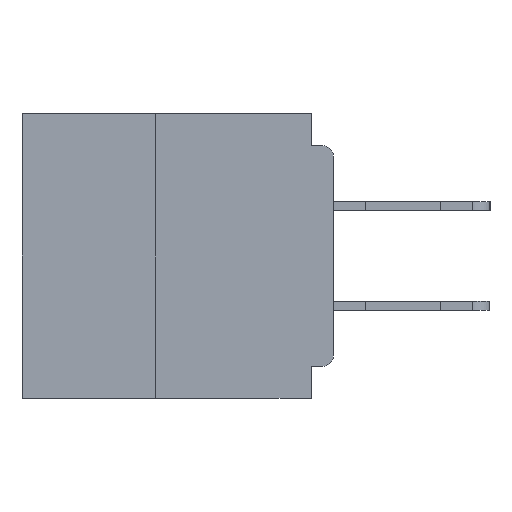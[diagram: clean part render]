
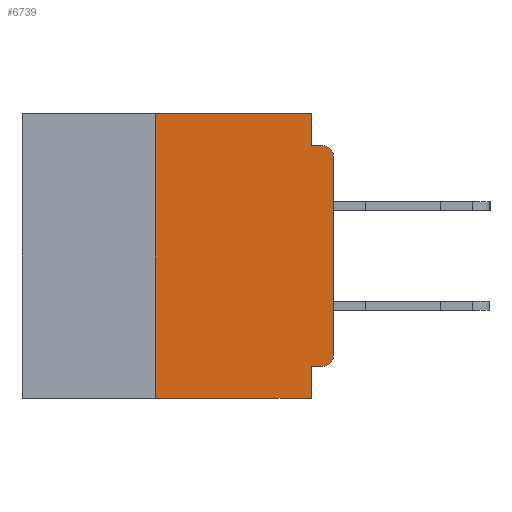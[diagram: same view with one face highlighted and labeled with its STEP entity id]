
A CAD part, left-side view. The second image highlights one B-rep face of the part: STEP entity #6739.
In plain terms, the highlighted planar face has unit normal (-1, 0, 0).
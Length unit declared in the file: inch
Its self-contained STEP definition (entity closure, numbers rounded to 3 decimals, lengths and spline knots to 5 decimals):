
#289 = AXIS2_PLACEMENT_3D ( 'NONE', #23680, #23636, #23599 ) ;
#902 = EDGE_CURVE ( 'NONE', #31502, #34823, #28456, .T. ) ;
#967 = DIRECTION ( 'NONE',  ( 0., -1., 0. ) ) ;
#1004 = FACE_OUTER_BOUND ( 'NONE', #19015, .T. ) ;
#1348 = EDGE_CURVE ( 'NONE', #32231, #15883, #28927, .T. ) ;
#1712 = ORIENTED_EDGE ( 'NONE', *, *, #23833, .F. ) ;
#2177 = LINE ( 'NONE', #33978, #9064 ) ;
#2724 = CARTESIAN_POINT ( 'NONE',  ( 0., 0.015, -0.355 ) ) ;
#2748 = VECTOR ( 'NONE', #9800, 39.37008 ) ;
#3122 = CARTESIAN_POINT ( 'NONE',  ( 0., 0.031, -0.045 ) ) ;
#3628 = EDGE_CURVE ( 'NONE', #30829, #5075, #4797, .T. ) ;
#3635 = VERTEX_POINT ( 'NONE', #24005 ) ;
#3698 = CARTESIAN_POINT ( 'NONE',  ( 0., 0.437, 0. ) ) ;
#3938 = CARTESIAN_POINT ( 'NONE',  ( 0., 0., -0.045 ) ) ;
#4179 = CIRCLE ( 'NONE', #33812, 0.015 ) ;
#4310 = EDGE_CURVE ( 'NONE', #5075, #3635, #10366, .T. ) ;
#4797 = CIRCLE ( 'NONE', #289, 0.015 ) ;
#5075 = VERTEX_POINT ( 'NONE', #13107 ) ;
#5424 = CARTESIAN_POINT ( 'NONE',  ( 0., 0.25, -0.4 ) ) ;
#5605 = DIRECTION ( 'NONE',  ( -1., 0., 0. ) ) ;
#5881 = VECTOR ( 'NONE', #26564, 39.37008 ) ;
#6739 = ADVANCED_FACE ( 'NONE', ( #1004 ), #11468, .F. ) ;
#8107 = VERTEX_POINT ( 'NONE', #34473 ) ;
#8190 = DIRECTION ( 'NONE',  ( 0., 1., 0. ) ) ;
#8366 = DIRECTION ( 'NONE',  ( 0., 0., 1. ) ) ;
#8437 = CARTESIAN_POINT ( 'NONE',  ( 0., 0.25, -0.4 ) ) ;
#8696 = DIRECTION ( 'NONE',  ( 0., 0., 1. ) ) ;
#9035 = CARTESIAN_POINT ( 'NONE',  ( 0., 0., 0. ) ) ;
#9064 = VECTOR ( 'NONE', #11214, 39.37008 ) ;
#9800 = DIRECTION ( 'NONE',  ( 0., -1., 0. ) ) ;
#10366 = LINE ( 'NONE', #9035, #11311 ) ;
#10683 = AXIS2_PLACEMENT_3D ( 'NONE', #11421, #11381, #11342 ) ;
#11214 = DIRECTION ( 'NONE',  ( 0., 0., -1. ) ) ;
#11311 = VECTOR ( 'NONE', #8696, 39.37008 ) ;
#11342 = DIRECTION ( 'NONE',  ( 0., 0., -1. ) ) ;
#11381 = DIRECTION ( 'NONE',  ( 1., 0., 0. ) ) ;
#11421 = CARTESIAN_POINT ( 'NONE',  ( 0., 0.437, 0. ) ) ;
#11468 = PLANE ( 'NONE',  #10683 ) ;
#11872 = EDGE_CURVE ( 'NONE', #3635, #8107, #4179, .T. ) ;
#12154 = VERTEX_POINT ( 'NONE', #24176 ) ;
#12159 = EDGE_CURVE ( 'NONE', #15883, #8107, #18328, .T. ) ;
#12610 = VECTOR ( 'NONE', #8366, 39.37008 ) ;
#13107 = CARTESIAN_POINT ( 'NONE',  ( 0., 0., -0.34 ) ) ;
#14173 = VERTEX_POINT ( 'NONE', #33707 ) ;
#14464 = LINE ( 'NONE', #5424, #12610 ) ;
#14592 = ORIENTED_EDGE ( 'NONE', *, *, #31884, .F. ) ;
#14683 = VECTOR ( 'NONE', #967, 39.37008 ) ;
#15883 = VERTEX_POINT ( 'NONE', #3122 ) ;
#16240 = VECTOR ( 'NONE', #8190, 39.37008 ) ;
#18328 = LINE ( 'NONE', #3938, #2748 ) ;
#19015 = EDGE_LOOP ( 'NONE', ( #25302, #32853, #19529, #27104, #36316, #14592, #29814, #23963, #1712, #25765 ) ) ;
#19529 = ORIENTED_EDGE ( 'NONE', *, *, #12159, .F. ) ;
#20847 = VECTOR ( 'NONE', #29407, 39.37008 ) ;
#21674 = EDGE_CURVE ( 'NONE', #14173, #34823, #2177, .T. ) ;
#22941 = CARTESIAN_POINT ( 'NONE',  ( 0., 0.015, -0.06 ) ) ;
#23599 = DIRECTION ( 'NONE',  ( 0., 0., -1. ) ) ;
#23636 = DIRECTION ( 'NONE',  ( -1., 0., 0. ) ) ;
#23680 = CARTESIAN_POINT ( 'NONE',  ( 0., 0.015, -0.34 ) ) ;
#23833 = EDGE_CURVE ( 'NONE', #30829, #14173, #31366, .T. ) ;
#23963 = ORIENTED_EDGE ( 'NONE', *, *, #21674, .F. ) ;
#24005 = CARTESIAN_POINT ( 'NONE',  ( 0., 0., -0.06 ) ) ;
#24176 = CARTESIAN_POINT ( 'NONE',  ( 0., 0.25, 0. ) ) ;
#25302 = ORIENTED_EDGE ( 'NONE', *, *, #4310, .T. ) ;
#25765 = ORIENTED_EDGE ( 'NONE', *, *, #3628, .T. ) ;
#25838 = DIRECTION ( 'NONE',  ( 0., 0., -1. ) ) ;
#26564 = DIRECTION ( 'NONE',  ( 0., 0., -1. ) ) ;
#26689 = CARTESIAN_POINT ( 'NONE',  ( 0., 0.031, 0. ) ) ;
#27104 = ORIENTED_EDGE ( 'NONE', *, *, #1348, .F. ) ;
#28398 = CARTESIAN_POINT ( 'NONE',  ( 0., 0., -0.355 ) ) ;
#28456 = LINE ( 'NONE', #36431, #20847 ) ;
#28530 = CARTESIAN_POINT ( 'NONE',  ( 0., 0.031, -0.4 ) ) ;
#28927 = LINE ( 'NONE', #26689, #5881 ) ;
#29407 = DIRECTION ( 'NONE',  ( 0., -1., 0. ) ) ;
#29814 = ORIENTED_EDGE ( 'NONE', *, *, #902, .T. ) ;
#29897 = LINE ( 'NONE', #3698, #14683 ) ;
#30140 = CARTESIAN_POINT ( 'NONE',  ( 0., 0.031, 0. ) ) ;
#30829 = VERTEX_POINT ( 'NONE', #2724 ) ;
#31366 = LINE ( 'NONE', #28398, #16240 ) ;
#31502 = VERTEX_POINT ( 'NONE', #8437 ) ;
#31884 = EDGE_CURVE ( 'NONE', #31502, #12154, #14464, .T. ) ;
#32231 = VERTEX_POINT ( 'NONE', #30140 ) ;
#32853 = ORIENTED_EDGE ( 'NONE', *, *, #11872, .T. ) ;
#33707 = CARTESIAN_POINT ( 'NONE',  ( 0., 0.031, -0.355 ) ) ;
#33812 = AXIS2_PLACEMENT_3D ( 'NONE', #22941, #5605, #25838 ) ;
#33978 = CARTESIAN_POINT ( 'NONE',  ( 0., 0.031, -0.4 ) ) ;
#34473 = CARTESIAN_POINT ( 'NONE',  ( 0., 0.015, -0.045 ) ) ;
#34823 = VERTEX_POINT ( 'NONE', #28530 ) ;
#35692 = EDGE_CURVE ( 'NONE', #12154, #32231, #29897, .T. ) ;
#36316 = ORIENTED_EDGE ( 'NONE', *, *, #35692, .F. ) ;
#36431 = CARTESIAN_POINT ( 'NONE',  ( 0., 0.437, -0.4 ) ) ;
